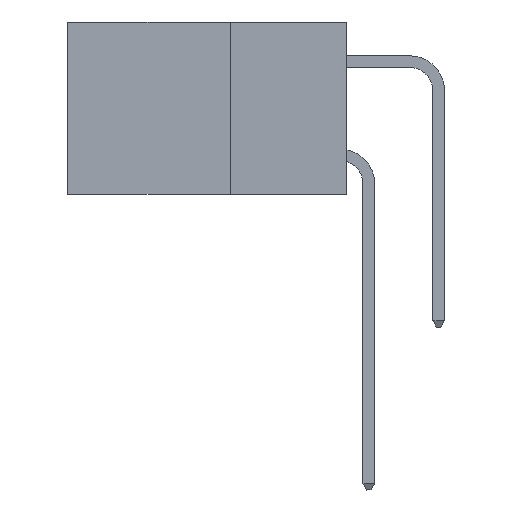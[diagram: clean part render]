
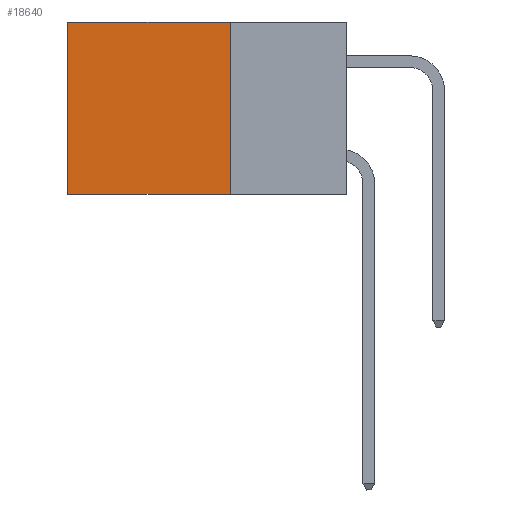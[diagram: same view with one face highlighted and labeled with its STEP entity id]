
A CAD part, left-side view. The second image highlights one B-rep face of the part: STEP entity #18640.
In plain terms, the highlighted planar face has unit normal (-1, 0, 0).
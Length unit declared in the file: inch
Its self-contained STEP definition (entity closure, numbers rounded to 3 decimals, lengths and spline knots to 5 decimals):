
#628 = VERTEX_POINT ( 'NONE', #16008 ) ;
#1912 = EDGE_CURVE ( 'NONE', #628, #13095, #18659, .T. ) ;
#1919 = CARTESIAN_POINT ( 'NONE',  ( 0.2875, 0.25, 0. ) ) ;
#2076 = CARTESIAN_POINT ( 'NONE',  ( 0.2875, 0.25, 0. ) ) ;
#2921 = VECTOR ( 'NONE', #7902, 39.37008 ) ;
#3417 = CARTESIAN_POINT ( 'NONE',  ( 0.2875, 0.6, 0. ) ) ;
#3480 = EDGE_CURVE ( 'NONE', #13095, #9683, #8232, .T. ) ;
#4027 = DIRECTION ( 'NONE',  ( 0., 1., 0. ) ) ;
#4111 = VECTOR ( 'NONE', #12362, 39.37008 ) ;
#4904 = DIRECTION ( 'NONE',  ( 1., 0., 0. ) ) ;
#5031 = DIRECTION ( 'NONE',  ( 0., 0., -1. ) ) ;
#5330 = VECTOR ( 'NONE', #5031, 39.37008 ) ;
#6843 = VERTEX_POINT ( 'NONE', #3417 ) ;
#7483 = EDGE_LOOP ( 'NONE', ( #9536, #18311, #25191, #9946 ) ) ;
#7902 = DIRECTION ( 'NONE',  ( 0., 0., -1. ) ) ;
#8232 = LINE ( 'NONE', #20323, #4111 ) ;
#9536 = ORIENTED_EDGE ( 'NONE', *, *, #10428, .T. ) ;
#9683 = VERTEX_POINT ( 'NONE', #22928 ) ;
#9923 = DIRECTION ( 'NONE',  ( 0., 0., -1. ) ) ;
#9946 = ORIENTED_EDGE ( 'NONE', *, *, #11986, .T. ) ;
#10312 = CARTESIAN_POINT ( 'NONE',  ( 0.2875, 0.25, 0. ) ) ;
#10428 = EDGE_CURVE ( 'NONE', #6843, #9683, #16657, .T. ) ;
#10759 = PLANE ( 'NONE',  #24408 ) ;
#11986 = EDGE_CURVE ( 'NONE', #628, #6843, #23631, .T. ) ;
#12362 = DIRECTION ( 'NONE',  ( 0., 1., 0. ) ) ;
#13095 = VERTEX_POINT ( 'NONE', #21311 ) ;
#16008 = CARTESIAN_POINT ( 'NONE',  ( 0.2875, 0.25, 0. ) ) ;
#16657 = LINE ( 'NONE', #23351, #5330 ) ;
#17646 = VECTOR ( 'NONE', #4027, 39.37008 ) ;
#18311 = ORIENTED_EDGE ( 'NONE', *, *, #3480, .F. ) ;
#18640 = ADVANCED_FACE ( 'NONE', ( #24901 ), #10759, .F. ) ;
#18659 = LINE ( 'NONE', #2076, #2921 ) ;
#20323 = CARTESIAN_POINT ( 'NONE',  ( 0.2875, 0.25, -0.37 ) ) ;
#21311 = CARTESIAN_POINT ( 'NONE',  ( 0.2875, 0.25, -0.37 ) ) ;
#22928 = CARTESIAN_POINT ( 'NONE',  ( 0.2875, 0.6, -0.37 ) ) ;
#23351 = CARTESIAN_POINT ( 'NONE',  ( 0.2875, 0.6, 0. ) ) ;
#23631 = LINE ( 'NONE', #1919, #17646 ) ;
#24408 = AXIS2_PLACEMENT_3D ( 'NONE', #10312, #4904, #9923 ) ;
#24901 = FACE_OUTER_BOUND ( 'NONE', #7483, .T. ) ;
#25191 = ORIENTED_EDGE ( 'NONE', *, *, #1912, .F. ) ;
